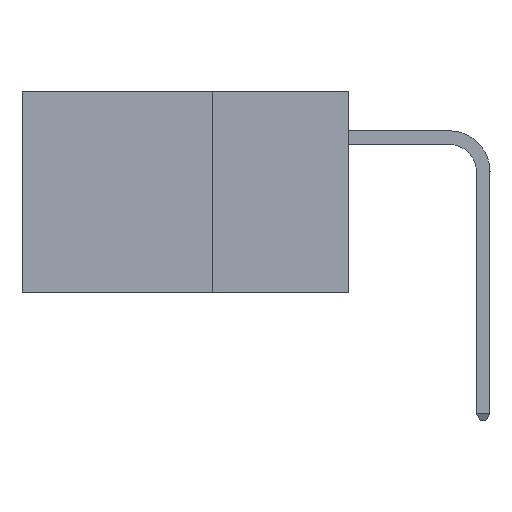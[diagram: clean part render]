
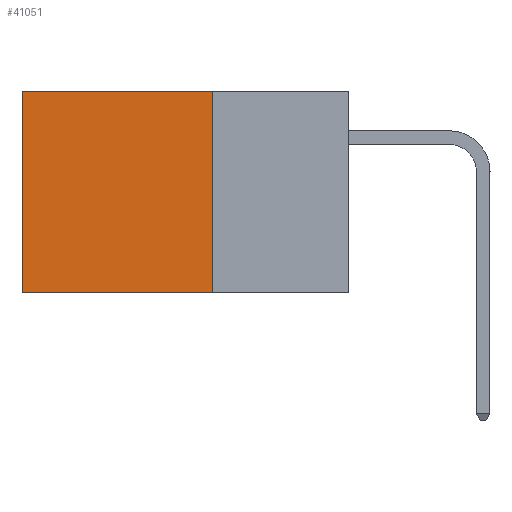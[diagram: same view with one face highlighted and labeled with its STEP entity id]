
A CAD part, left-side view. The second image highlights one B-rep face of the part: STEP entity #41051.
In plain terms, the highlighted planar face has unit normal (-1, 0, 0).
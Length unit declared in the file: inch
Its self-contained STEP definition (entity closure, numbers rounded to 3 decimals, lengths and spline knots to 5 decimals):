
#715 = PLANE ( 'NONE',  #16376 ) ;
#1723 = CARTESIAN_POINT ( 'NONE',  ( 0.2875, 0.25, -0.37 ) ) ;
#2065 = VERTEX_POINT ( 'NONE', #30652 ) ;
#3909 = EDGE_LOOP ( 'NONE', ( #23146, #28238, #37414, #40519 ) ) ;
#4144 = DIRECTION ( 'NONE',  ( 1., 0., 0. ) ) ;
#5421 = LINE ( 'NONE', #1723, #21352 ) ;
#5467 = VERTEX_POINT ( 'NONE', #36647 ) ;
#6178 = EDGE_CURVE ( 'NONE', #6734, #36851, #43272, .T. ) ;
#6734 = VERTEX_POINT ( 'NONE', #42703 ) ;
#7583 = LINE ( 'NONE', #28787, #8638 ) ;
#7860 = EDGE_CURVE ( 'NONE', #2065, #6734, #7583, .T. ) ;
#8638 = VECTOR ( 'NONE', #15100, 39.37008 ) ;
#12408 = CARTESIAN_POINT ( 'NONE',  ( 0.2875, 0.6, -0.37 ) ) ;
#14175 = CARTESIAN_POINT ( 'NONE',  ( 0.2875, 0.25, 0. ) ) ;
#15100 = DIRECTION ( 'NONE',  ( 0., 1., 0. ) ) ;
#16376 = AXIS2_PLACEMENT_3D ( 'NONE', #14175, #4144, #27849 ) ;
#16664 = CARTESIAN_POINT ( 'NONE',  ( 0.2875, 0.6, 0. ) ) ;
#20686 = EDGE_CURVE ( 'NONE', #2065, #5467, #39570, .T. ) ;
#21352 = VECTOR ( 'NONE', #32237, 39.37008 ) ;
#23146 = ORIENTED_EDGE ( 'NONE', *, *, #6178, .T. ) ;
#23524 = DIRECTION ( 'NONE',  ( 0., 0., -1. ) ) ;
#27849 = DIRECTION ( 'NONE',  ( 0., 0., -1. ) ) ;
#28238 = ORIENTED_EDGE ( 'NONE', *, *, #32951, .F. ) ;
#28787 = CARTESIAN_POINT ( 'NONE',  ( 0.2875, 0.25, 0. ) ) ;
#30498 = VECTOR ( 'NONE', #39797, 39.37008 ) ;
#30652 = CARTESIAN_POINT ( 'NONE',  ( 0.2875, 0.25, 0. ) ) ;
#32237 = DIRECTION ( 'NONE',  ( 0., 1., 0. ) ) ;
#32951 = EDGE_CURVE ( 'NONE', #5467, #36851, #5421, .T. ) ;
#36647 = CARTESIAN_POINT ( 'NONE',  ( 0.2875, 0.25, -0.37 ) ) ;
#36851 = VERTEX_POINT ( 'NONE', #12408 ) ;
#37414 = ORIENTED_EDGE ( 'NONE', *, *, #20686, .F. ) ;
#39570 = LINE ( 'NONE', #43355, #30498 ) ;
#39797 = DIRECTION ( 'NONE',  ( 0., 0., -1. ) ) ;
#40519 = ORIENTED_EDGE ( 'NONE', *, *, #7860, .T. ) ;
#40577 = FACE_OUTER_BOUND ( 'NONE', #3909, .T. ) ;
#41051 = ADVANCED_FACE ( 'NONE', ( #40577 ), #715, .F. ) ;
#42229 = VECTOR ( 'NONE', #23524, 39.37008 ) ;
#42703 = CARTESIAN_POINT ( 'NONE',  ( 0.2875, 0.6, 0. ) ) ;
#43272 = LINE ( 'NONE', #16664, #42229 ) ;
#43355 = CARTESIAN_POINT ( 'NONE',  ( 0.2875, 0.25, 0. ) ) ;
